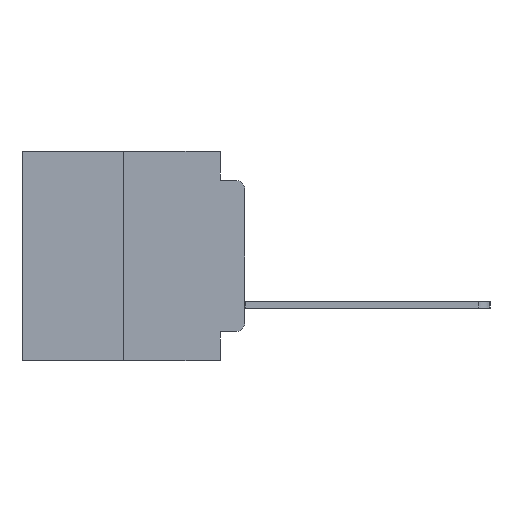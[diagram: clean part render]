
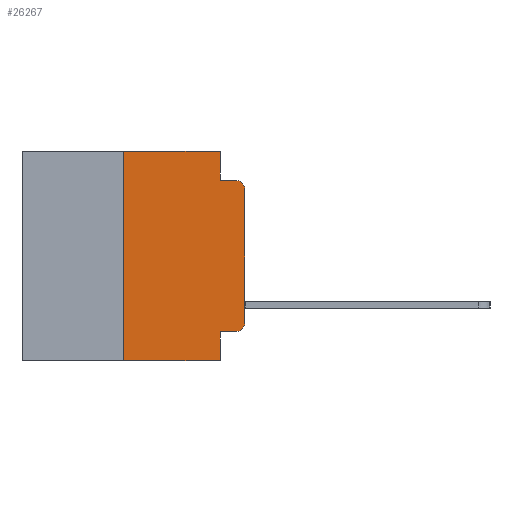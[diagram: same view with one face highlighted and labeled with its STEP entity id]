
A CAD part, left-side view. The second image highlights one B-rep face of the part: STEP entity #26267.
In plain terms, the highlighted planar face has unit normal (-1, 0, 0).
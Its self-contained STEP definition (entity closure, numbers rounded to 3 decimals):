
#304 = AXIS2_PLACEMENT_3D ( 'NONE', #9696, #18726, #7505 ) ;
#720 = VERTEX_POINT ( 'NONE', #23088 ) ;
#988 = VECTOR ( 'NONE', #9914, 1000. ) ;
#1096 = CARTESIAN_POINT ( 'NONE',  ( -75.603, 1.295, 0. ) ) ;
#1435 = CARTESIAN_POINT ( 'NONE',  ( -75.603, 0., -3.467 ) ) ;
#2997 = ORIENTED_EDGE ( 'NONE', *, *, #27163, .F. ) ;
#3082 = EDGE_CURVE ( 'NONE', #3269, #720, #15990, .T. ) ;
#3269 = VERTEX_POINT ( 'NONE', #12316 ) ;
#3332 = CARTESIAN_POINT ( 'NONE',  ( -75.603, 0., 3.467 ) ) ;
#4281 = DIRECTION ( 'NONE',  ( 0., -1., 0. ) ) ;
#4367 = VECTOR ( 'NONE', #6014, 1000. ) ;
#4750 = ORIENTED_EDGE ( 'NONE', *, *, #27263, .F. ) ;
#4905 = CARTESIAN_POINT ( 'NONE',  ( -75.603, 11.684, 5.486 ) ) ;
#5217 = VERTEX_POINT ( 'NONE', #1435 ) ;
#5243 = FACE_OUTER_BOUND ( 'NONE', #13192, .T. ) ;
#5516 = LINE ( 'NONE', #15425, #18547 ) ;
#5523 = ORIENTED_EDGE ( 'NONE', *, *, #7235, .F. ) ;
#6014 = DIRECTION ( 'NONE',  ( 0., 0., 1. ) ) ;
#6043 = EDGE_CURVE ( 'NONE', #7200, #8192, #5516, .T. ) ;
#6124 = CARTESIAN_POINT ( 'NONE',  ( -75.603, 1.295, 0. ) ) ;
#6290 = CARTESIAN_POINT ( 'NONE',  ( -75.603, 1.295, 3.975 ) ) ;
#6304 = DIRECTION ( 'NONE',  ( 0., 0., -1. ) ) ;
#6761 = DIRECTION ( 'NONE',  ( 0., -1., 0. ) ) ;
#7077 = CIRCLE ( 'NONE', #11976, 0.508 ) ;
#7200 = VERTEX_POINT ( 'NONE', #21600 ) ;
#7235 = EDGE_CURVE ( 'NONE', #22284, #16000, #16449, .T. ) ;
#7269 = DIRECTION ( 'NONE',  ( 0., 0., -1. ) ) ;
#7505 = DIRECTION ( 'NONE',  ( 0., 0., -1. ) ) ;
#8192 = VERTEX_POINT ( 'NONE', #27986 ) ;
#8785 = DIRECTION ( 'NONE',  ( 0., -1., 0. ) ) ;
#9112 = DIRECTION ( 'NONE',  ( 0., 0., -1. ) ) ;
#9696 = CARTESIAN_POINT ( 'NONE',  ( -75.603, 0.508, 3.467 ) ) ;
#9914 = DIRECTION ( 'NONE',  ( 0., 0., 1. ) ) ;
#9953 = EDGE_CURVE ( 'NONE', #28123, #23955, #28039, .T. ) ;
#10375 = EDGE_CURVE ( 'NONE', #5217, #28123, #27980, .T. ) ;
#10788 = ORIENTED_EDGE ( 'NONE', *, *, #3082, .T. ) ;
#11035 = ORIENTED_EDGE ( 'NONE', *, *, #27368, .T. ) ;
#11508 = ORIENTED_EDGE ( 'NONE', *, *, #15100, .F. ) ;
#11538 = LINE ( 'NONE', #6124, #16715 ) ;
#11615 = DIRECTION ( 'NONE',  ( 0., 0., -1. ) ) ;
#11698 = VECTOR ( 'NONE', #7269, 1000. ) ;
#11976 = AXIS2_PLACEMENT_3D ( 'NONE', #18260, #15768, #11615 ) ;
#12220 = VERTEX_POINT ( 'NONE', #6290 ) ;
#12316 = CARTESIAN_POINT ( 'NONE',  ( -75.603, 1.295, -3.975 ) ) ;
#12387 = LINE ( 'NONE', #1096, #11698 ) ;
#13084 = CARTESIAN_POINT ( 'NONE',  ( -75.603, 1.295, 3.975 ) ) ;
#13192 = EDGE_LOOP ( 'NONE', ( #10788, #11035, #20424, #16875, #4750, #11508, #5523, #27316, #18217, #2997 ) ) ;
#13227 = DIRECTION ( 'NONE',  ( 0., -1., 0. ) ) ;
#14296 = LINE ( 'NONE', #13084, #27996 ) ;
#15100 = EDGE_CURVE ( 'NONE', #16000, #12220, #12387, .T. ) ;
#15425 = CARTESIAN_POINT ( 'NONE',  ( -75.603, 11.684, -5.486 ) ) ;
#15674 = CARTESIAN_POINT ( 'NONE',  ( -75.603, 1.295, -3.975 ) ) ;
#15768 = DIRECTION ( 'NONE',  ( -1., 0., 0. ) ) ;
#15831 = PLANE ( 'NONE',  #18058 ) ;
#15990 = LINE ( 'NONE', #15674, #28302 ) ;
#16000 = VERTEX_POINT ( 'NONE', #17473 ) ;
#16449 = LINE ( 'NONE', #17577, #17138 ) ;
#16715 = VECTOR ( 'NONE', #6304, 1000. ) ;
#16875 = ORIENTED_EDGE ( 'NONE', *, *, #9953, .T. ) ;
#17138 = VECTOR ( 'NONE', #6761, 1000. ) ;
#17473 = CARTESIAN_POINT ( 'NONE',  ( -75.603, 1.295, 5.486 ) ) ;
#17577 = CARTESIAN_POINT ( 'NONE',  ( -75.603, 11.684, 5.486 ) ) ;
#18058 = AXIS2_PLACEMENT_3D ( 'NONE', #4905, #19862, #9112 ) ;
#18217 = ORIENTED_EDGE ( 'NONE', *, *, #6043, .T. ) ;
#18260 = CARTESIAN_POINT ( 'NONE',  ( -75.603, 0.508, -3.467 ) ) ;
#18429 = EDGE_CURVE ( 'NONE', #7200, #22284, #21154, .T. ) ;
#18547 = VECTOR ( 'NONE', #13227, 1000. ) ;
#18726 = DIRECTION ( 'NONE',  ( -1., 0., 0. ) ) ;
#19862 = DIRECTION ( 'NONE',  ( 1., 0., 0. ) ) ;
#20424 = ORIENTED_EDGE ( 'NONE', *, *, #10375, .T. ) ;
#21154 = LINE ( 'NONE', #24885, #988 ) ;
#21328 = CARTESIAN_POINT ( 'NONE',  ( -75.603, 0., 5.486 ) ) ;
#21600 = CARTESIAN_POINT ( 'NONE',  ( -75.603, 6.35, -5.486 ) ) ;
#22284 = VERTEX_POINT ( 'NONE', #26885 ) ;
#22499 = CARTESIAN_POINT ( 'NONE',  ( -75.603, 0.508, 3.975 ) ) ;
#23088 = CARTESIAN_POINT ( 'NONE',  ( -75.603, 0.508, -3.975 ) ) ;
#23955 = VERTEX_POINT ( 'NONE', #22499 ) ;
#24885 = CARTESIAN_POINT ( 'NONE',  ( -75.603, 6.35, -5.486 ) ) ;
#26267 = ADVANCED_FACE ( 'NONE', ( #5243 ), #15831, .F. ) ;
#26885 = CARTESIAN_POINT ( 'NONE',  ( -75.603, 6.35, 5.486 ) ) ;
#27163 = EDGE_CURVE ( 'NONE', #3269, #8192, #11538, .T. ) ;
#27263 = EDGE_CURVE ( 'NONE', #12220, #23955, #14296, .T. ) ;
#27316 = ORIENTED_EDGE ( 'NONE', *, *, #18429, .F. ) ;
#27368 = EDGE_CURVE ( 'NONE', #720, #5217, #7077, .T. ) ;
#27980 = LINE ( 'NONE', #21328, #4367 ) ;
#27986 = CARTESIAN_POINT ( 'NONE',  ( -75.603, 1.295, -5.486 ) ) ;
#27996 = VECTOR ( 'NONE', #8785, 1000. ) ;
#28039 = CIRCLE ( 'NONE', #304, 0.508 ) ;
#28123 = VERTEX_POINT ( 'NONE', #3332 ) ;
#28302 = VECTOR ( 'NONE', #4281, 1000. ) ;
